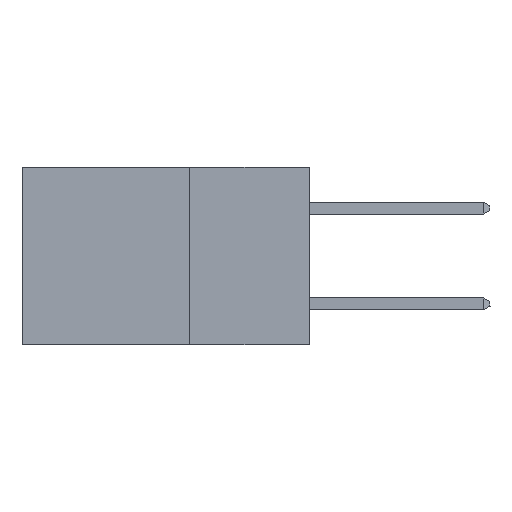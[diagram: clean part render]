
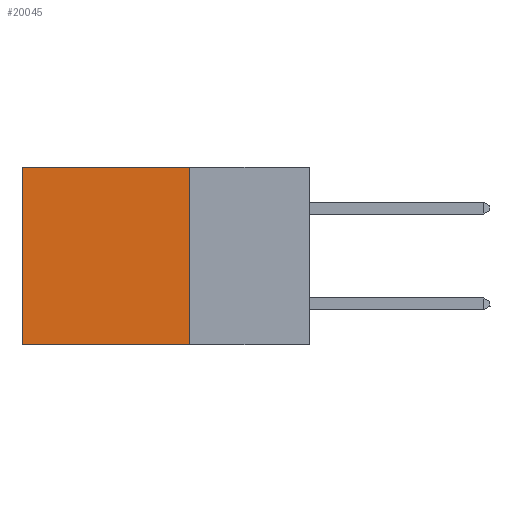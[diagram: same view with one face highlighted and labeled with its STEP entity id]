
A CAD part, left-side view. The second image highlights one B-rep face of the part: STEP entity #20045.
In plain terms, the highlighted planar face has unit normal (-1, 0, 0).
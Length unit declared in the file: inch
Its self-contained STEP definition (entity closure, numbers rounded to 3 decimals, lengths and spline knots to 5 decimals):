
#1275 = VECTOR ( 'NONE', #21131, 39.37008 ) ;
#1346 = VECTOR ( 'NONE', #6305, 39.37008 ) ;
#1579 = PLANE ( 'NONE',  #3200 ) ;
#2557 = VERTEX_POINT ( 'NONE', #19233 ) ;
#3200 = AXIS2_PLACEMENT_3D ( 'NONE', #14302, #21878, #13946 ) ;
#3880 = LINE ( 'NONE', #21125, #1346 ) ;
#4921 = VERTEX_POINT ( 'NONE', #9713 ) ;
#4989 = LINE ( 'NONE', #18651, #9771 ) ;
#6305 = DIRECTION ( 'NONE',  ( 0., 0., -1. ) ) ;
#6707 = LINE ( 'NONE', #15133, #20753 ) ;
#7098 = CARTESIAN_POINT ( 'NONE',  ( 0.2875, 0.25, 0. ) ) ;
#7233 = EDGE_CURVE ( 'NONE', #4921, #25774, #4989, .T. ) ;
#8665 = CARTESIAN_POINT ( 'NONE',  ( 0.2875, 0.6, -0.37 ) ) ;
#9246 = ORIENTED_EDGE ( 'NONE', *, *, #19547, .T. ) ;
#9713 = CARTESIAN_POINT ( 'NONE',  ( 0.2875, 0.25, -0.37 ) ) ;
#9771 = VECTOR ( 'NONE', #22721, 39.37008 ) ;
#12811 = CARTESIAN_POINT ( 'NONE',  ( 0.2875, 0.25, 0. ) ) ;
#13946 = DIRECTION ( 'NONE',  ( 0., 0., -1. ) ) ;
#14302 = CARTESIAN_POINT ( 'NONE',  ( 0.2875, 0.25, 0. ) ) ;
#14489 = EDGE_CURVE ( 'NONE', #24785, #4921, #3880, .T. ) ;
#14849 = ORIENTED_EDGE ( 'NONE', *, *, #14489, .F. ) ;
#15005 = ORIENTED_EDGE ( 'NONE', *, *, #19826, .T. ) ;
#15133 = CARTESIAN_POINT ( 'NONE',  ( 0.2875, 0.6, 0. ) ) ;
#17816 = LINE ( 'NONE', #12811, #1275 ) ;
#18077 = EDGE_LOOP ( 'NONE', ( #9246, #22619, #14849, #15005 ) ) ;
#18651 = CARTESIAN_POINT ( 'NONE',  ( 0.2875, 0.25, -0.37 ) ) ;
#19064 = DIRECTION ( 'NONE',  ( 0., 0., -1. ) ) ;
#19119 = FACE_OUTER_BOUND ( 'NONE', #18077, .T. ) ;
#19233 = CARTESIAN_POINT ( 'NONE',  ( 0.2875, 0.6, 0. ) ) ;
#19547 = EDGE_CURVE ( 'NONE', #2557, #25774, #6707, .T. ) ;
#19826 = EDGE_CURVE ( 'NONE', #24785, #2557, #17816, .T. ) ;
#20045 = ADVANCED_FACE ( 'NONE', ( #19119 ), #1579, .F. ) ;
#20753 = VECTOR ( 'NONE', #19064, 39.37008 ) ;
#21125 = CARTESIAN_POINT ( 'NONE',  ( 0.2875, 0.25, 0. ) ) ;
#21131 = DIRECTION ( 'NONE',  ( 0., 1., 0. ) ) ;
#21878 = DIRECTION ( 'NONE',  ( 1., 0., 0. ) ) ;
#22619 = ORIENTED_EDGE ( 'NONE', *, *, #7233, .F. ) ;
#22721 = DIRECTION ( 'NONE',  ( 0., 1., 0. ) ) ;
#24785 = VERTEX_POINT ( 'NONE', #7098 ) ;
#25774 = VERTEX_POINT ( 'NONE', #8665 ) ;
